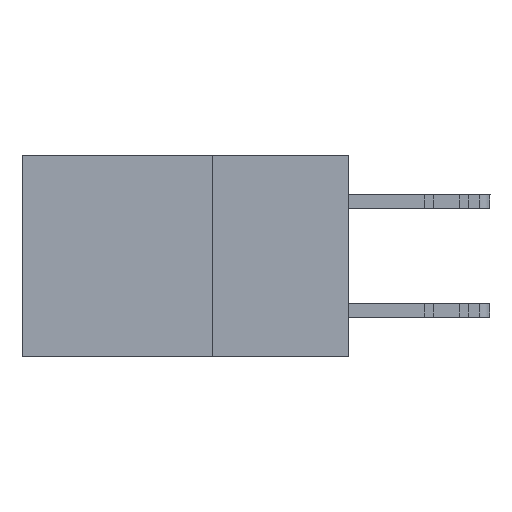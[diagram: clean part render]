
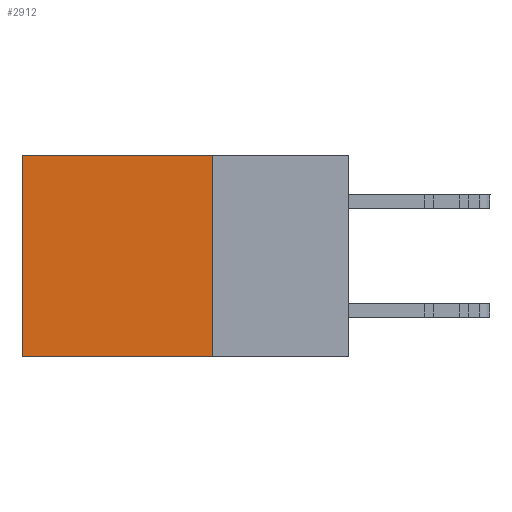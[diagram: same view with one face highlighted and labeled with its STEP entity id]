
A CAD part, left-side view. The second image highlights one B-rep face of the part: STEP entity #2912.
In plain terms, the highlighted planar face has unit normal (-1, 0, 0).
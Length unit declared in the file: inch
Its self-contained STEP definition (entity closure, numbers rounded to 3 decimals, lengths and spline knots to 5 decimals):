
#258 = DIRECTION ( 'NONE',  ( 0., 1., 0. ) ) ;
#785 = LINE ( 'NONE', #14106, #21733 ) ;
#1963 = VERTEX_POINT ( 'NONE', #12616 ) ;
#2389 = EDGE_LOOP ( 'NONE', ( #7542, #10932, #23215, #7744 ) ) ;
#2912 = ADVANCED_FACE ( 'NONE', ( #24124 ), #21414, .F. ) ;
#6219 = LINE ( 'NONE', #25951, #27330 ) ;
#7542 = ORIENTED_EDGE ( 'NONE', *, *, #23645, .T. ) ;
#7744 = ORIENTED_EDGE ( 'NONE', *, *, #17947, .T. ) ;
#8630 = DIRECTION ( 'NONE',  ( 0., 1., 0. ) ) ;
#10500 = VERTEX_POINT ( 'NONE', #13793 ) ;
#10932 = ORIENTED_EDGE ( 'NONE', *, *, #18182, .F. ) ;
#12616 = CARTESIAN_POINT ( 'NONE',  ( 0.298, 0.25, -0.37 ) ) ;
#13169 = CARTESIAN_POINT ( 'NONE',  ( 0.298, 0.25, 0. ) ) ;
#13793 = CARTESIAN_POINT ( 'NONE',  ( 0.298, 0.6, 0. ) ) ;
#14106 = CARTESIAN_POINT ( 'NONE',  ( 0.298, 0.25, 0. ) ) ;
#14149 = LINE ( 'NONE', #23017, #19380 ) ;
#15148 = LINE ( 'NONE', #23871, #24020 ) ;
#15326 = EDGE_CURVE ( 'NONE', #24916, #1963, #785, .T. ) ;
#17382 = DIRECTION ( 'NONE',  ( 0., 0., -1. ) ) ;
#17947 = EDGE_CURVE ( 'NONE', #24916, #10500, #14149, .T. ) ;
#18182 = EDGE_CURVE ( 'NONE', #1963, #25644, #15148, .T. ) ;
#19092 = DIRECTION ( 'NONE',  ( 1., 0., 0. ) ) ;
#19380 = VECTOR ( 'NONE', #258, 39.37008 ) ;
#20793 = DIRECTION ( 'NONE',  ( 0., 0., -1. ) ) ;
#21414 = PLANE ( 'NONE',  #21840 ) ;
#21733 = VECTOR ( 'NONE', #20793, 39.37008 ) ;
#21840 = AXIS2_PLACEMENT_3D ( 'NONE', #28608, #19092, #21948 ) ;
#21948 = DIRECTION ( 'NONE',  ( 0., 0., -1. ) ) ;
#23017 = CARTESIAN_POINT ( 'NONE',  ( 0.298, 0.25, 0. ) ) ;
#23215 = ORIENTED_EDGE ( 'NONE', *, *, #15326, .F. ) ;
#23645 = EDGE_CURVE ( 'NONE', #10500, #25644, #6219, .T. ) ;
#23871 = CARTESIAN_POINT ( 'NONE',  ( 0.298, 0.25, -0.37 ) ) ;
#24020 = VECTOR ( 'NONE', #8630, 39.37008 ) ;
#24124 = FACE_OUTER_BOUND ( 'NONE', #2389, .T. ) ;
#24916 = VERTEX_POINT ( 'NONE', #13169 ) ;
#25644 = VERTEX_POINT ( 'NONE', #27618 ) ;
#25951 = CARTESIAN_POINT ( 'NONE',  ( 0.298, 0.6, 0. ) ) ;
#27330 = VECTOR ( 'NONE', #17382, 39.37008 ) ;
#27618 = CARTESIAN_POINT ( 'NONE',  ( 0.298, 0.6, -0.37 ) ) ;
#28608 = CARTESIAN_POINT ( 'NONE',  ( 0.298, 0.25, 0. ) ) ;
